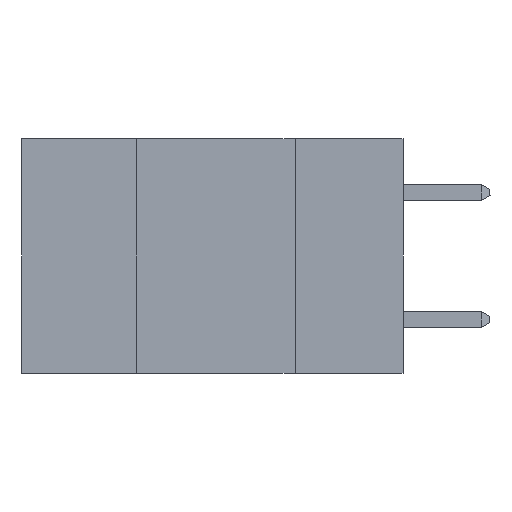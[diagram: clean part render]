
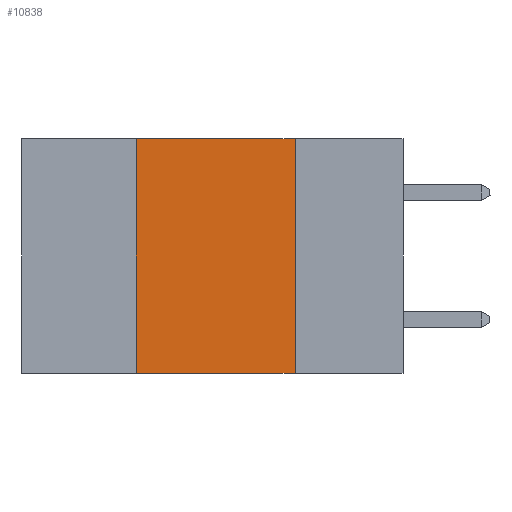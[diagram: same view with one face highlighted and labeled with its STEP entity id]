
A CAD part, left-side view. The second image highlights one B-rep face of the part: STEP entity #10838.
In plain terms, the highlighted planar face has unit normal (-1, 0, 0).
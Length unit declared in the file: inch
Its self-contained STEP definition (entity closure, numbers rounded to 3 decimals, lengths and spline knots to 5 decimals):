
#86 = VERTEX_POINT ( 'NONE', #4196 ) ;
#382 = EDGE_LOOP ( 'NONE', ( #15515, #10991, #1577, #593 ) ) ;
#529 = DIRECTION ( 'NONE',  ( 0., 0., 1. ) ) ;
#553 = LINE ( 'NONE', #7064, #14829 ) ;
#593 = ORIENTED_EDGE ( 'NONE', *, *, #15895, .T. ) ;
#1577 = ORIENTED_EDGE ( 'NONE', *, *, #16556, .F. ) ;
#1725 = VERTEX_POINT ( 'NONE', #12160 ) ;
#1803 = EDGE_CURVE ( 'NONE', #8373, #1725, #553, .T. ) ;
#1995 = CARTESIAN_POINT ( 'NONE',  ( 0., 0.6, -0.37 ) ) ;
#2020 = CARTESIAN_POINT ( 'NONE',  ( 0., 0.42, 0. ) ) ;
#2043 = DIRECTION ( 'NONE',  ( 1., 0., 0. ) ) ;
#4143 = CARTESIAN_POINT ( 'NONE',  ( 0., 0.6, 0. ) ) ;
#4196 = CARTESIAN_POINT ( 'NONE',  ( 0., 0.42, 0. ) ) ;
#4229 = DIRECTION ( 'NONE',  ( 0., -1., 0. ) ) ;
#4429 = PLANE ( 'NONE',  #8230 ) ;
#4671 = VERTEX_POINT ( 'NONE', #8100 ) ;
#5109 = VECTOR ( 'NONE', #4229, 39.37008 ) ;
#5632 = LINE ( 'NONE', #4143, #5109 ) ;
#6342 = VECTOR ( 'NONE', #529, 39.37008 ) ;
#7064 = CARTESIAN_POINT ( 'NONE',  ( 0., 0.17, 0. ) ) ;
#7128 = CARTESIAN_POINT ( 'NONE',  ( 0., 0.17, 0. ) ) ;
#7350 = DIRECTION ( 'NONE',  ( 0., -1., 0. ) ) ;
#8100 = CARTESIAN_POINT ( 'NONE',  ( 0., 0.42, -0.37 ) ) ;
#8230 = AXIS2_PLACEMENT_3D ( 'NONE', #16654, #2043, #15429 ) ;
#8373 = VERTEX_POINT ( 'NONE', #7128 ) ;
#9763 = LINE ( 'NONE', #2020, #6342 ) ;
#9942 = EDGE_CURVE ( 'NONE', #86, #8373, #5632, .T. ) ;
#10838 = ADVANCED_FACE ( 'NONE', ( #16414 ), #4429, .F. ) ;
#10991 = ORIENTED_EDGE ( 'NONE', *, *, #9942, .F. ) ;
#12160 = CARTESIAN_POINT ( 'NONE',  ( 0., 0.17, -0.37 ) ) ;
#12324 = DIRECTION ( 'NONE',  ( 0., 0., -1. ) ) ;
#14829 = VECTOR ( 'NONE', #12324, 39.37008 ) ;
#15429 = DIRECTION ( 'NONE',  ( 0., 0., -1. ) ) ;
#15515 = ORIENTED_EDGE ( 'NONE', *, *, #1803, .F. ) ;
#15524 = VECTOR ( 'NONE', #7350, 39.37008 ) ;
#15895 = EDGE_CURVE ( 'NONE', #4671, #1725, #16694, .T. ) ;
#16414 = FACE_OUTER_BOUND ( 'NONE', #382, .T. ) ;
#16556 = EDGE_CURVE ( 'NONE', #4671, #86, #9763, .T. ) ;
#16654 = CARTESIAN_POINT ( 'NONE',  ( 0., 0.6, 0. ) ) ;
#16694 = LINE ( 'NONE', #1995, #15524 ) ;
